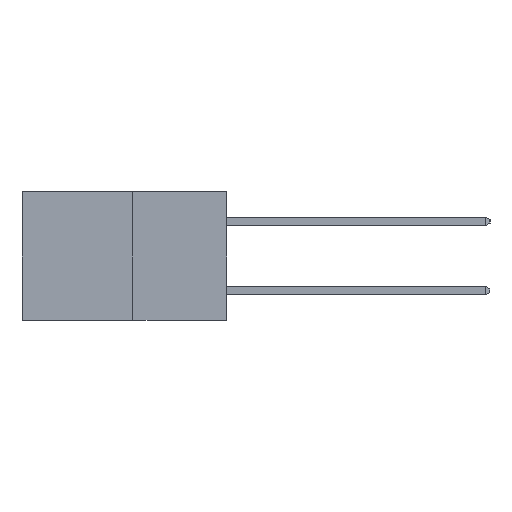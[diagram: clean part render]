
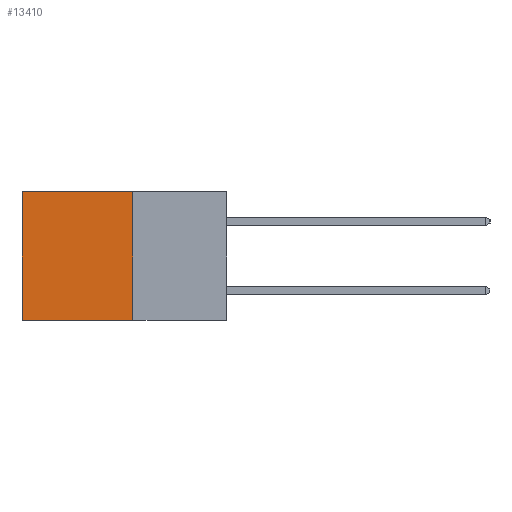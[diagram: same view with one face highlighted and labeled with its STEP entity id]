
A CAD part, left-side view. The second image highlights one B-rep face of the part: STEP entity #13410.
In plain terms, the highlighted planar face has unit normal (-1, 0, 0).
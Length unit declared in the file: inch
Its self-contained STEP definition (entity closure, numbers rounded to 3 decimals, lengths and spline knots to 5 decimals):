
#487 = AXIS2_PLACEMENT_3D ( 'NONE', #17022, #18915, #7603 ) ;
#1896 = ORIENTED_EDGE ( 'NONE', *, *, #24208, .F. ) ;
#2080 = FACE_OUTER_BOUND ( 'NONE', #4793, .T. ) ;
#3316 = CARTESIAN_POINT ( 'NONE',  ( 0.277, 0.59, -0.37 ) ) ;
#3784 = PLANE ( 'NONE',  #487 ) ;
#4178 = VECTOR ( 'NONE', #7463, 39.37008 ) ;
#4257 = ORIENTED_EDGE ( 'NONE', *, *, #23334, .F. ) ;
#4793 = EDGE_LOOP ( 'NONE', ( #9882, #4257, #1896, #18733 ) ) ;
#5022 = CARTESIAN_POINT ( 'NONE',  ( 0.277, 0.59, 0. ) ) ;
#7463 = DIRECTION ( 'NONE',  ( 0., 0., -1. ) ) ;
#7603 = DIRECTION ( 'NONE',  ( 0., 0., -1. ) ) ;
#7797 = VECTOR ( 'NONE', #10539, 39.37008 ) ;
#8113 = VERTEX_POINT ( 'NONE', #3316 ) ;
#8884 = CARTESIAN_POINT ( 'NONE',  ( 0.277, 0.27, 0. ) ) ;
#9701 = CARTESIAN_POINT ( 'NONE',  ( 0.277, 0.27, -0.37 ) ) ;
#9779 = VECTOR ( 'NONE', #19996, 39.37008 ) ;
#9861 = VERTEX_POINT ( 'NONE', #5022 ) ;
#9882 = ORIENTED_EDGE ( 'NONE', *, *, #17020, .T. ) ;
#10539 = DIRECTION ( 'NONE',  ( 0., 1., 0. ) ) ;
#11660 = DIRECTION ( 'NONE',  ( 0., 0., -1. ) ) ;
#12290 = LINE ( 'NONE', #21759, #7797 ) ;
#12488 = EDGE_CURVE ( 'NONE', #22861, #9861, #12290, .T. ) ;
#13410 = ADVANCED_FACE ( 'NONE', ( #2080 ), #3784, .F. ) ;
#13879 = VERTEX_POINT ( 'NONE', #18313 ) ;
#15148 = VECTOR ( 'NONE', #11660, 39.37008 ) ;
#15397 = LINE ( 'NONE', #9701, #15148 ) ;
#17020 = EDGE_CURVE ( 'NONE', #9861, #8113, #23539, .T. ) ;
#17022 = CARTESIAN_POINT ( 'NONE',  ( 0.277, 0.27, -0.37 ) ) ;
#18118 = CARTESIAN_POINT ( 'NONE',  ( 0.277, 0.27, -0.37 ) ) ;
#18313 = CARTESIAN_POINT ( 'NONE',  ( 0.277, 0.27, -0.37 ) ) ;
#18733 = ORIENTED_EDGE ( 'NONE', *, *, #12488, .T. ) ;
#18764 = CARTESIAN_POINT ( 'NONE',  ( 0.277, 0.59, -0.37 ) ) ;
#18915 = DIRECTION ( 'NONE',  ( 1., 0., 0. ) ) ;
#19796 = LINE ( 'NONE', #18118, #9779 ) ;
#19996 = DIRECTION ( 'NONE',  ( 0., 1., 0. ) ) ;
#21759 = CARTESIAN_POINT ( 'NONE',  ( 0.277, 0.27, 0. ) ) ;
#22861 = VERTEX_POINT ( 'NONE', #8884 ) ;
#23334 = EDGE_CURVE ( 'NONE', #13879, #8113, #19796, .T. ) ;
#23539 = LINE ( 'NONE', #18764, #4178 ) ;
#24208 = EDGE_CURVE ( 'NONE', #22861, #13879, #15397, .T. ) ;
